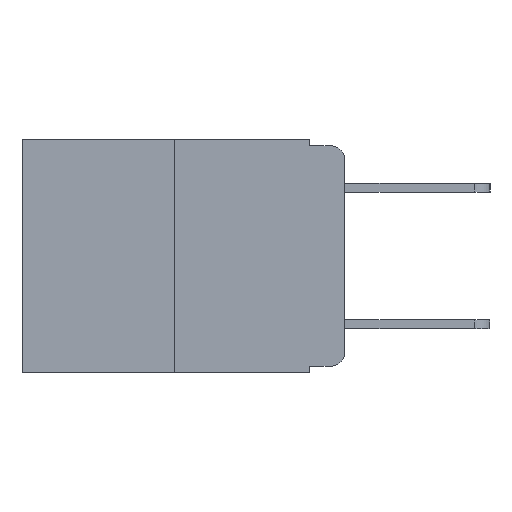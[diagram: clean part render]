
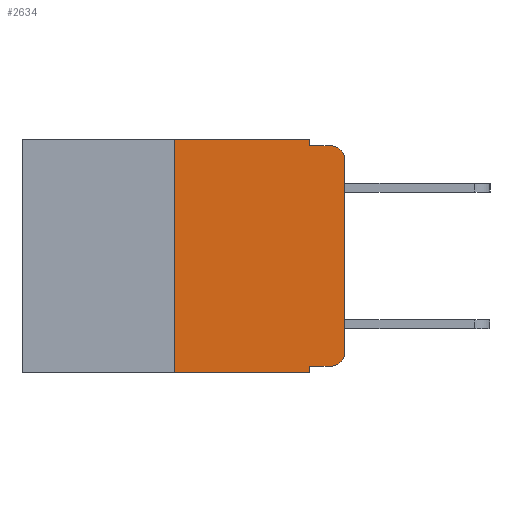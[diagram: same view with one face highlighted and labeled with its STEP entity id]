
A CAD part, left-side view. The second image highlights one B-rep face of the part: STEP entity #2634.
In plain terms, the highlighted planar face has unit normal (-1, 0, 0).
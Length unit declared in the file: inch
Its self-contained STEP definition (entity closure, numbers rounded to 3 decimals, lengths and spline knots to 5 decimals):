
#21 = VERTEX_POINT ( 'NONE', #9818 ) ;
#542 = EDGE_CURVE ( 'NONE', #21, #4019, #10918, .T. ) ;
#729 = ORIENTED_EDGE ( 'NONE', *, *, #542, .F. ) ;
#855 = CARTESIAN_POINT ( 'NONE',  ( 0., 0.051, -0.333 ) ) ;
#868 = VERTEX_POINT ( 'NONE', #11665 ) ;
#907 = CARTESIAN_POINT ( 'NONE',  ( 0., 0.25, 0. ) ) ;
#962 = LINE ( 'NONE', #2111, #3873 ) ;
#1268 = VERTEX_POINT ( 'NONE', #12126 ) ;
#1385 = CIRCLE ( 'NONE', #11963, 0.02 ) ;
#1690 = CARTESIAN_POINT ( 'NONE',  ( 0., 0.051, 0. ) ) ;
#1871 = DIRECTION ( 'NONE',  ( -1., 0., 0. ) ) ;
#1997 = EDGE_CURVE ( 'NONE', #7579, #2291, #1385, .T. ) ;
#2058 = CARTESIAN_POINT ( 'NONE',  ( 0., 0.473, 0. ) ) ;
#2111 = CARTESIAN_POINT ( 'NONE',  ( 0., 0.473, 0. ) ) ;
#2149 = LINE ( 'NONE', #10422, #12766 ) ;
#2242 = EDGE_CURVE ( 'NONE', #4019, #2291, #2149, .T. ) ;
#2251 = AXIS2_PLACEMENT_3D ( 'NONE', #2058, #6698, #6633 ) ;
#2291 = VERTEX_POINT ( 'NONE', #3472 ) ;
#2306 = EDGE_CURVE ( 'NONE', #6902, #9721, #6511, .T. ) ;
#2318 = FACE_OUTER_BOUND ( 'NONE', #7527, .T. ) ;
#2625 = EDGE_CURVE ( 'NONE', #6270, #1268, #13126, .T. ) ;
#2627 = EDGE_CURVE ( 'NONE', #6902, #868, #5812, .T. ) ;
#2634 = ADVANCED_FACE ( 'NONE', ( #2318 ), #10536, .F. ) ;
#2762 = DIRECTION ( 'NONE',  ( 0., 0., -1. ) ) ;
#3183 = VERTEX_POINT ( 'NONE', #11897 ) ;
#3334 = EDGE_CURVE ( 'NONE', #868, #3183, #8170, .T. ) ;
#3472 = CARTESIAN_POINT ( 'NONE',  ( 0., 0.02, -0.01 ) ) ;
#3742 = DIRECTION ( 'NONE',  ( 0., -1., 0. ) ) ;
#3832 = EDGE_CURVE ( 'NONE', #6270, #9721, #13554, .T. ) ;
#3873 = VECTOR ( 'NONE', #7757, 39.37008 ) ;
#3875 = ORIENTED_EDGE ( 'NONE', *, *, #2306, .F. ) ;
#4019 = VERTEX_POINT ( 'NONE', #11008 ) ;
#4029 = ORIENTED_EDGE ( 'NONE', *, *, #8776, .F. ) ;
#4127 = CARTESIAN_POINT ( 'NONE',  ( 0., 0.051, 0. ) ) ;
#4149 = DIRECTION ( 'NONE',  ( 0., 0., -1. ) ) ;
#4766 = EDGE_CURVE ( 'NONE', #3183, #7579, #10186, .T. ) ;
#4942 = CARTESIAN_POINT ( 'NONE',  ( 0., 0., -0.03 ) ) ;
#5115 = CARTESIAN_POINT ( 'NONE',  ( 0., 0.051, -0.343 ) ) ;
#5586 = DIRECTION ( 'NONE',  ( 0., -1., 0. ) ) ;
#5657 = ORIENTED_EDGE ( 'NONE', *, *, #4766, .T. ) ;
#5812 = LINE ( 'NONE', #12058, #12876 ) ;
#6270 = VERTEX_POINT ( 'NONE', #13243 ) ;
#6328 = ORIENTED_EDGE ( 'NONE', *, *, #2242, .F. ) ;
#6511 = LINE ( 'NONE', #1690, #8942 ) ;
#6633 = DIRECTION ( 'NONE',  ( 0., 0., -1. ) ) ;
#6698 = DIRECTION ( 'NONE',  ( 1., 0., 0. ) ) ;
#6902 = VERTEX_POINT ( 'NONE', #855 ) ;
#7181 = VECTOR ( 'NONE', #11853, 39.37008 ) ;
#7527 = EDGE_LOOP ( 'NONE', ( #5657, #13250, #6328, #729, #4029, #10848, #8945, #3875, #12249, #12770 ) ) ;
#7579 = VERTEX_POINT ( 'NONE', #4942 ) ;
#7757 = DIRECTION ( 'NONE',  ( 0., -1., 0. ) ) ;
#8170 = CIRCLE ( 'NONE', #8606, 0.02 ) ;
#8589 = CARTESIAN_POINT ( 'NONE',  ( 0., 0.02, -0.313 ) ) ;
#8606 = AXIS2_PLACEMENT_3D ( 'NONE', #8589, #1871, #9627 ) ;
#8712 = CARTESIAN_POINT ( 'NONE',  ( 0., 0.473, -0.343 ) ) ;
#8776 = EDGE_CURVE ( 'NONE', #1268, #21, #962, .T. ) ;
#8942 = VECTOR ( 'NONE', #4149, 39.37008 ) ;
#8945 = ORIENTED_EDGE ( 'NONE', *, *, #3832, .T. ) ;
#9627 = DIRECTION ( 'NONE',  ( 0., 0., -1. ) ) ;
#9721 = VERTEX_POINT ( 'NONE', #5115 ) ;
#9818 = CARTESIAN_POINT ( 'NONE',  ( 0., 0.051, 0. ) ) ;
#10186 = LINE ( 'NONE', #10961, #7181 ) ;
#10422 = CARTESIAN_POINT ( 'NONE',  ( 0., 0.051, -0.01 ) ) ;
#10536 = PLANE ( 'NONE',  #2251 ) ;
#10634 = VECTOR ( 'NONE', #2762, 39.37008 ) ;
#10848 = ORIENTED_EDGE ( 'NONE', *, *, #2625, .F. ) ;
#10918 = LINE ( 'NONE', #4127, #10634 ) ;
#10961 = CARTESIAN_POINT ( 'NONE',  ( 0., 0., 0. ) ) ;
#11008 = CARTESIAN_POINT ( 'NONE',  ( 0., 0.051, -0.01 ) ) ;
#11378 = DIRECTION ( 'NONE',  ( 0., 0., 1. ) ) ;
#11665 = CARTESIAN_POINT ( 'NONE',  ( 0., 0.02, -0.333 ) ) ;
#11853 = DIRECTION ( 'NONE',  ( 0., 0., 1. ) ) ;
#11897 = CARTESIAN_POINT ( 'NONE',  ( 0., 0., -0.313 ) ) ;
#11963 = AXIS2_PLACEMENT_3D ( 'NONE', #12497, #12482, #12199 ) ;
#12058 = CARTESIAN_POINT ( 'NONE',  ( 0., 0.051, -0.333 ) ) ;
#12126 = CARTESIAN_POINT ( 'NONE',  ( 0., 0.25, 0. ) ) ;
#12199 = DIRECTION ( 'NONE',  ( 0., 0., -1. ) ) ;
#12249 = ORIENTED_EDGE ( 'NONE', *, *, #2627, .T. ) ;
#12482 = DIRECTION ( 'NONE',  ( -1., 0., 0. ) ) ;
#12497 = CARTESIAN_POINT ( 'NONE',  ( 0., 0.02, -0.03 ) ) ;
#12766 = VECTOR ( 'NONE', #5586, 39.37008 ) ;
#12770 = ORIENTED_EDGE ( 'NONE', *, *, #3334, .T. ) ;
#12876 = VECTOR ( 'NONE', #3742, 39.37008 ) ;
#13126 = LINE ( 'NONE', #907, #13381 ) ;
#13236 = DIRECTION ( 'NONE',  ( 0., -1., 0. ) ) ;
#13243 = CARTESIAN_POINT ( 'NONE',  ( 0., 0.25, -0.343 ) ) ;
#13250 = ORIENTED_EDGE ( 'NONE', *, *, #1997, .T. ) ;
#13281 = VECTOR ( 'NONE', #13236, 39.37008 ) ;
#13381 = VECTOR ( 'NONE', #11378, 39.37008 ) ;
#13554 = LINE ( 'NONE', #8712, #13281 ) ;
